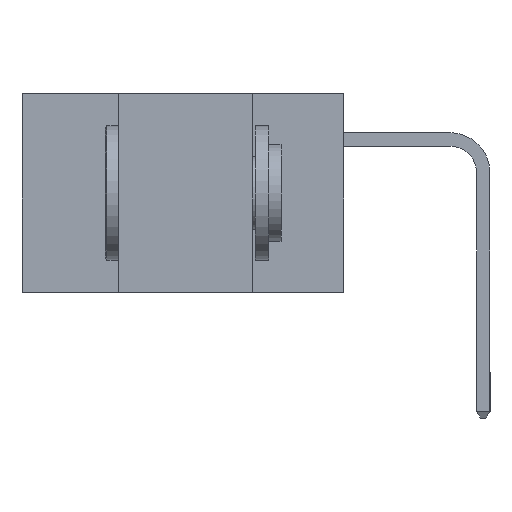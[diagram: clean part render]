
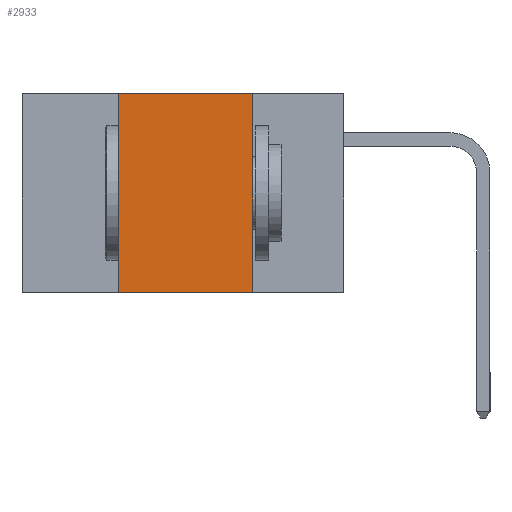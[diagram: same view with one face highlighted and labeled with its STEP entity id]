
A CAD part, left-side view. The second image highlights one B-rep face of the part: STEP entity #2933.
In plain terms, the highlighted planar face has unit normal (-1, 0, 0).
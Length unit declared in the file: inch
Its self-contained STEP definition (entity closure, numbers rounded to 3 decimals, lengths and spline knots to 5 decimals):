
#345 = EDGE_CURVE ( 'NONE', #10516, #14715, #10667, .T. ) ;
#1773 = CARTESIAN_POINT ( 'NONE',  ( 0., 0.17, -0.37 ) ) ;
#1833 = ORIENTED_EDGE ( 'NONE', *, *, #2953, .F. ) ;
#2514 = VECTOR ( 'NONE', #5425, 39.37008 ) ;
#2933 = ADVANCED_FACE ( 'NONE', ( #17297 ), #3689, .F. ) ;
#2953 = EDGE_CURVE ( 'NONE', #13627, #10516, #17537, .T. ) ;
#3074 = DIRECTION ( 'NONE',  ( 0., -1., 0. ) ) ;
#3259 = CARTESIAN_POINT ( 'NONE',  ( 0., 0.42, 0. ) ) ;
#3689 = PLANE ( 'NONE',  #5905 ) ;
#4445 = LINE ( 'NONE', #14823, #2514 ) ;
#5425 = DIRECTION ( 'NONE',  ( 0., 0., -1. ) ) ;
#5862 = VECTOR ( 'NONE', #3074, 39.37008 ) ;
#5905 = AXIS2_PLACEMENT_3D ( 'NONE', #14373, #14249, #8275 ) ;
#6399 = CARTESIAN_POINT ( 'NONE',  ( 0., 0.6, 0. ) ) ;
#7852 = CARTESIAN_POINT ( 'NONE',  ( 0., 0.6, -0.37 ) ) ;
#8275 = DIRECTION ( 'NONE',  ( 0., 0., -1. ) ) ;
#8955 = EDGE_LOOP ( 'NONE', ( #12027, #11006, #1833, #16197 ) ) ;
#9554 = CARTESIAN_POINT ( 'NONE',  ( 0., 0.42, 0. ) ) ;
#10516 = VERTEX_POINT ( 'NONE', #3259 ) ;
#10667 = LINE ( 'NONE', #6399, #15691 ) ;
#11006 = ORIENTED_EDGE ( 'NONE', *, *, #345, .F. ) ;
#11019 = DIRECTION ( 'NONE',  ( 0., -1., 0. ) ) ;
#11099 = DIRECTION ( 'NONE',  ( 0., 0., 1. ) ) ;
#11629 = LINE ( 'NONE', #7852, #5862 ) ;
#12027 = ORIENTED_EDGE ( 'NONE', *, *, #14123, .F. ) ;
#12253 = VECTOR ( 'NONE', #11099, 39.37008 ) ;
#12796 = CARTESIAN_POINT ( 'NONE',  ( 0., 0.17, 0. ) ) ;
#13627 = VERTEX_POINT ( 'NONE', #19252 ) ;
#14123 = EDGE_CURVE ( 'NONE', #14715, #17680, #4445, .T. ) ;
#14249 = DIRECTION ( 'NONE',  ( 1., 0., 0. ) ) ;
#14373 = CARTESIAN_POINT ( 'NONE',  ( 0., 0.6, 0. ) ) ;
#14715 = VERTEX_POINT ( 'NONE', #12796 ) ;
#14823 = CARTESIAN_POINT ( 'NONE',  ( 0., 0.17, 0. ) ) ;
#15691 = VECTOR ( 'NONE', #11019, 39.37008 ) ;
#16161 = EDGE_CURVE ( 'NONE', #13627, #17680, #11629, .T. ) ;
#16197 = ORIENTED_EDGE ( 'NONE', *, *, #16161, .T. ) ;
#17297 = FACE_OUTER_BOUND ( 'NONE', #8955, .T. ) ;
#17537 = LINE ( 'NONE', #9554, #12253 ) ;
#17680 = VERTEX_POINT ( 'NONE', #1773 ) ;
#19252 = CARTESIAN_POINT ( 'NONE',  ( 0., 0.42, -0.37 ) ) ;
